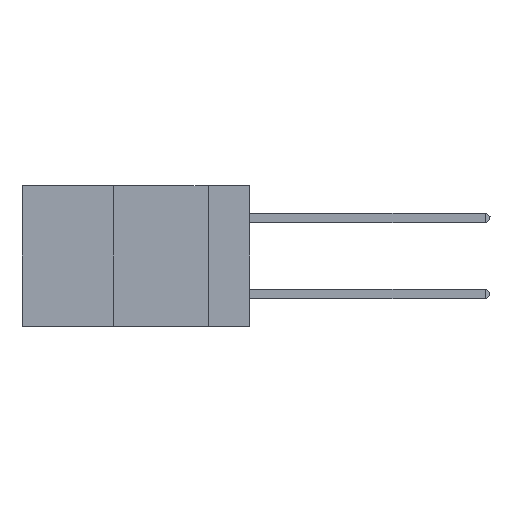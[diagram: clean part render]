
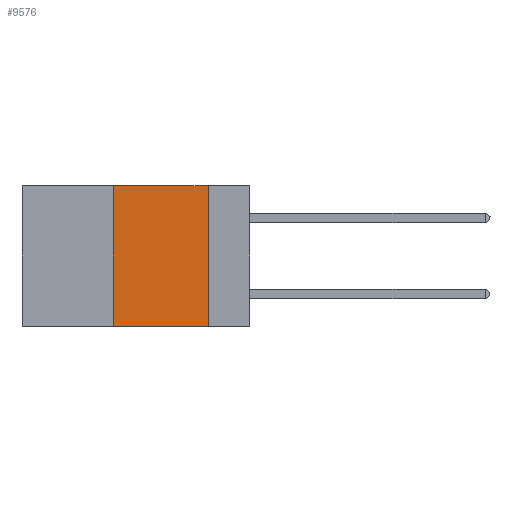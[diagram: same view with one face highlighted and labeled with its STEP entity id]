
A CAD part, left-side view. The second image highlights one B-rep face of the part: STEP entity #9576.
In plain terms, the highlighted planar face has unit normal (-1, 0, 0).
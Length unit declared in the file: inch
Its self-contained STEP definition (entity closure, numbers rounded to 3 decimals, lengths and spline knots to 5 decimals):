
#101 = ORIENTED_EDGE ( 'NONE', *, *, #1939, .F. ) ;
#122 = LINE ( 'NONE', #1351, #6868 ) ;
#690 = EDGE_LOOP ( 'NONE', ( #1026, #3767, #101, #5751 ) ) ;
#1026 = ORIENTED_EDGE ( 'NONE', *, *, #6798, .F. ) ;
#1044 = LINE ( 'NONE', #3743, #6220 ) ;
#1230 = VERTEX_POINT ( 'NONE', #9739 ) ;
#1351 = CARTESIAN_POINT ( 'NONE',  ( 0., 0.36, 0. ) ) ;
#1707 = CARTESIAN_POINT ( 'NONE',  ( 0., 0.11, -0.37 ) ) ;
#1939 = EDGE_CURVE ( 'NONE', #1230, #2606, #122, .T. ) ;
#1975 = PLANE ( 'NONE',  #8971 ) ;
#2606 = VERTEX_POINT ( 'NONE', #9383 ) ;
#3098 = DIRECTION ( 'NONE',  ( 0., -1., 0. ) ) ;
#3558 = EDGE_CURVE ( 'NONE', #2606, #7049, #10115, .T. ) ;
#3743 = CARTESIAN_POINT ( 'NONE',  ( 0., 0.11, 0. ) ) ;
#3767 = ORIENTED_EDGE ( 'NONE', *, *, #3558, .F. ) ;
#4389 = DIRECTION ( 'NONE',  ( 0., -1., 0. ) ) ;
#4794 = CARTESIAN_POINT ( 'NONE',  ( 0., 0.6, 0. ) ) ;
#5206 = VECTOR ( 'NONE', #3098, 39.37008 ) ;
#5652 = DIRECTION ( 'NONE',  ( 0., 0., -1. ) ) ;
#5696 = VERTEX_POINT ( 'NONE', #1707 ) ;
#5751 = ORIENTED_EDGE ( 'NONE', *, *, #9939, .T. ) ;
#5783 = CARTESIAN_POINT ( 'NONE',  ( 0., 0.11, 0. ) ) ;
#6220 = VECTOR ( 'NONE', #10696, 39.37008 ) ;
#6798 = EDGE_CURVE ( 'NONE', #7049, #5696, #1044, .T. ) ;
#6868 = VECTOR ( 'NONE', #9672, 39.37008 ) ;
#7049 = VERTEX_POINT ( 'NONE', #5783 ) ;
#7491 = CARTESIAN_POINT ( 'NONE',  ( 0., 0.6, 0. ) ) ;
#7873 = CARTESIAN_POINT ( 'NONE',  ( 0., 0.6, -0.37 ) ) ;
#8081 = LINE ( 'NONE', #7873, #10118 ) ;
#8971 = AXIS2_PLACEMENT_3D ( 'NONE', #4794, #10854, #5652 ) ;
#9383 = CARTESIAN_POINT ( 'NONE',  ( 0., 0.36, 0. ) ) ;
#9576 = ADVANCED_FACE ( 'NONE', ( #11286 ), #1975, .F. ) ;
#9672 = DIRECTION ( 'NONE',  ( 0., 0., 1. ) ) ;
#9739 = CARTESIAN_POINT ( 'NONE',  ( 0., 0.36, -0.37 ) ) ;
#9939 = EDGE_CURVE ( 'NONE', #1230, #5696, #8081, .T. ) ;
#10115 = LINE ( 'NONE', #7491, #5206 ) ;
#10118 = VECTOR ( 'NONE', #4389, 39.37008 ) ;
#10696 = DIRECTION ( 'NONE',  ( 0., 0., -1. ) ) ;
#10854 = DIRECTION ( 'NONE',  ( 1., 0., 0. ) ) ;
#11286 = FACE_OUTER_BOUND ( 'NONE', #690, .T. ) ;
